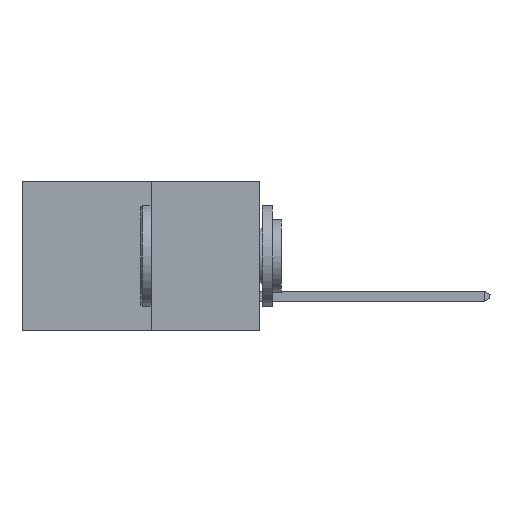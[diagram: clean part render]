
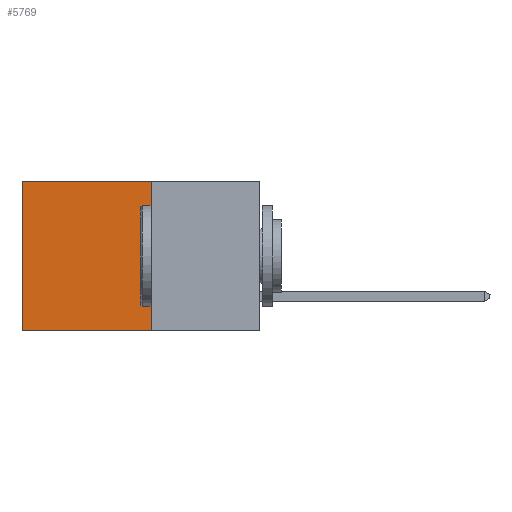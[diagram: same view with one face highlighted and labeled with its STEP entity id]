
A CAD part, left-side view. The second image highlights one B-rep face of the part: STEP entity #5769.
In plain terms, the highlighted planar face has unit normal (-1, 0, 0).
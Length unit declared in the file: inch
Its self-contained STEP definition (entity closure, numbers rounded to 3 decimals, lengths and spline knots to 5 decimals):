
#86 = VERTEX_POINT ( 'NONE', #26198 ) ;
#955 = LINE ( 'NONE', #13138, #6382 ) ;
#2075 = VECTOR ( 'NONE', #21363, 39.37008 ) ;
#2290 = CARTESIAN_POINT ( 'NONE',  ( 0.277, 0.59, -0.37 ) ) ;
#2580 = VERTEX_POINT ( 'NONE', #22590 ) ;
#3531 = LINE ( 'NONE', #19070, #2075 ) ;
#5769 = ADVANCED_FACE ( 'NONE', ( #6067 ), #17361, .F. ) ;
#6067 = FACE_OUTER_BOUND ( 'NONE', #7279, .T. ) ;
#6382 = VECTOR ( 'NONE', #22288, 39.37008 ) ;
#6387 = EDGE_CURVE ( 'NONE', #2580, #21107, #955, .T. ) ;
#6993 = LINE ( 'NONE', #19764, #26628 ) ;
#7279 = EDGE_LOOP ( 'NONE', ( #25622, #11123, #29285, #20758 ) ) ;
#8269 = CARTESIAN_POINT ( 'NONE',  ( 0.277, 0.27, -0.37 ) ) ;
#10899 = EDGE_CURVE ( 'NONE', #21107, #24754, #29492, .T. ) ;
#11123 = ORIENTED_EDGE ( 'NONE', *, *, #15935, .F. ) ;
#11722 = AXIS2_PLACEMENT_3D ( 'NONE', #8269, #12865, #28748 ) ;
#12865 = DIRECTION ( 'NONE',  ( 1., 0., 0. ) ) ;
#13138 = CARTESIAN_POINT ( 'NONE',  ( 0.277, 0.27, 0. ) ) ;
#15935 = EDGE_CURVE ( 'NONE', #86, #24754, #3531, .T. ) ;
#17361 = PLANE ( 'NONE',  #11722 ) ;
#19070 = CARTESIAN_POINT ( 'NONE',  ( 0.277, 0.27, -0.37 ) ) ;
#19764 = CARTESIAN_POINT ( 'NONE',  ( 0.277, 0.27, -0.37 ) ) ;
#20147 = EDGE_CURVE ( 'NONE', #2580, #86, #6993, .T. ) ;
#20758 = ORIENTED_EDGE ( 'NONE', *, *, #6387, .T. ) ;
#20776 = DIRECTION ( 'NONE',  ( 0., 0., -1. ) ) ;
#21107 = VERTEX_POINT ( 'NONE', #27199 ) ;
#21363 = DIRECTION ( 'NONE',  ( 0., 1., 0. ) ) ;
#22288 = DIRECTION ( 'NONE',  ( 0., 1., 0. ) ) ;
#22590 = CARTESIAN_POINT ( 'NONE',  ( 0.277, 0.27, 0. ) ) ;
#22973 = CARTESIAN_POINT ( 'NONE',  ( 0.277, 0.59, -0.37 ) ) ;
#24353 = DIRECTION ( 'NONE',  ( 0., 0., -1. ) ) ;
#24754 = VERTEX_POINT ( 'NONE', #2290 ) ;
#25622 = ORIENTED_EDGE ( 'NONE', *, *, #10899, .T. ) ;
#26198 = CARTESIAN_POINT ( 'NONE',  ( 0.277, 0.27, -0.37 ) ) ;
#26628 = VECTOR ( 'NONE', #24353, 39.37008 ) ;
#27199 = CARTESIAN_POINT ( 'NONE',  ( 0.277, 0.59, 0. ) ) ;
#28748 = DIRECTION ( 'NONE',  ( 0., 0., -1. ) ) ;
#28793 = VECTOR ( 'NONE', #20776, 39.37008 ) ;
#29285 = ORIENTED_EDGE ( 'NONE', *, *, #20147, .F. ) ;
#29492 = LINE ( 'NONE', #22973, #28793 ) ;
